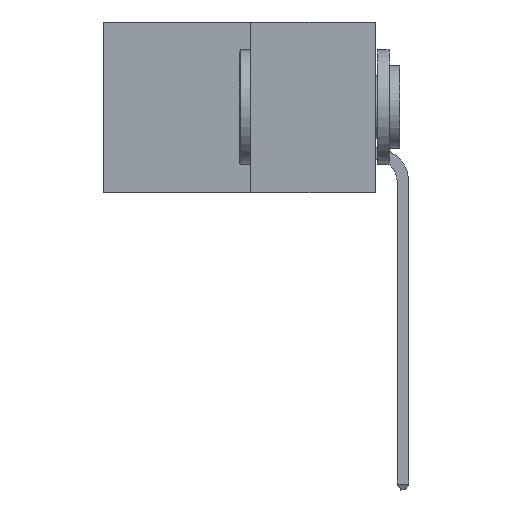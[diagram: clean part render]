
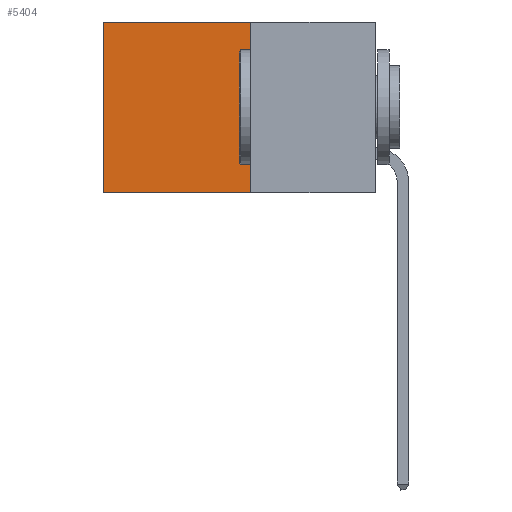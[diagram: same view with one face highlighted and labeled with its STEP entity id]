
A CAD part, left-side view. The second image highlights one B-rep face of the part: STEP entity #5404.
In plain terms, the highlighted planar face has unit normal (-1, 0, 0).
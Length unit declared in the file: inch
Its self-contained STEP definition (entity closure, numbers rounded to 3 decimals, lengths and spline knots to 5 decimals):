
#150 = EDGE_CURVE ( 'NONE', #18917, #17487, #13493, .T. ) ;
#573 = EDGE_CURVE ( 'NONE', #14104, #6826, #1869, .T. ) ;
#1776 = VECTOR ( 'NONE', #6837, 39.37008 ) ;
#1869 = LINE ( 'NONE', #18123, #13471 ) ;
#4515 = DIRECTION ( 'NONE',  ( 0., 0., -1. ) ) ;
#5404 = ADVANCED_FACE ( 'NONE', ( #25683 ), #15967, .F. ) ;
#6063 = DIRECTION ( 'NONE',  ( 0., 1., 0. ) ) ;
#6826 = VERTEX_POINT ( 'NONE', #8584 ) ;
#6837 = DIRECTION ( 'NONE',  ( 0., 0., -1. ) ) ;
#8584 = CARTESIAN_POINT ( 'NONE',  ( 0.277, 0.59, 0. ) ) ;
#9051 = CARTESIAN_POINT ( 'NONE',  ( 0.277, 0.27, -0.37 ) ) ;
#10400 = VECTOR ( 'NONE', #23733, 39.37008 ) ;
#13471 = VECTOR ( 'NONE', #15352, 39.37008 ) ;
#13493 = LINE ( 'NONE', #18417, #24855 ) ;
#14079 = LINE ( 'NONE', #27238, #1776 ) ;
#14104 = VERTEX_POINT ( 'NONE', #14251 ) ;
#14251 = CARTESIAN_POINT ( 'NONE',  ( 0.277, 0.27, 0. ) ) ;
#15352 = DIRECTION ( 'NONE',  ( 0., 1., 0. ) ) ;
#15733 = ORIENTED_EDGE ( 'NONE', *, *, #16852, .T. ) ;
#15967 = PLANE ( 'NONE',  #23384 ) ;
#16852 = EDGE_CURVE ( 'NONE', #6826, #17487, #14079, .T. ) ;
#16893 = CARTESIAN_POINT ( 'NONE',  ( 0.277, 0.27, -0.37 ) ) ;
#17487 = VERTEX_POINT ( 'NONE', #27104 ) ;
#18123 = CARTESIAN_POINT ( 'NONE',  ( 0.277, 0.27, 0. ) ) ;
#18269 = DIRECTION ( 'NONE',  ( 1., 0., 0. ) ) ;
#18311 = EDGE_CURVE ( 'NONE', #14104, #18917, #22519, .T. ) ;
#18417 = CARTESIAN_POINT ( 'NONE',  ( 0.277, 0.27, -0.37 ) ) ;
#18917 = VERTEX_POINT ( 'NONE', #19070 ) ;
#19070 = CARTESIAN_POINT ( 'NONE',  ( 0.277, 0.27, -0.37 ) ) ;
#20743 = ORIENTED_EDGE ( 'NONE', *, *, #150, .F. ) ;
#22238 = ORIENTED_EDGE ( 'NONE', *, *, #573, .T. ) ;
#22519 = LINE ( 'NONE', #16893, #10400 ) ;
#23384 = AXIS2_PLACEMENT_3D ( 'NONE', #9051, #18269, #4515 ) ;
#23733 = DIRECTION ( 'NONE',  ( 0., 0., -1. ) ) ;
#24331 = ORIENTED_EDGE ( 'NONE', *, *, #18311, .F. ) ;
#24855 = VECTOR ( 'NONE', #6063, 39.37008 ) ;
#25683 = FACE_OUTER_BOUND ( 'NONE', #27443, .T. ) ;
#27104 = CARTESIAN_POINT ( 'NONE',  ( 0.277, 0.59, -0.37 ) ) ;
#27238 = CARTESIAN_POINT ( 'NONE',  ( 0.277, 0.59, -0.37 ) ) ;
#27443 = EDGE_LOOP ( 'NONE', ( #15733, #20743, #24331, #22238 ) ) ;
